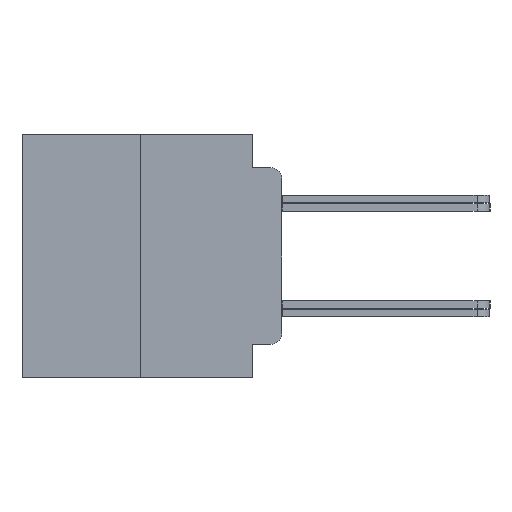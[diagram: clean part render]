
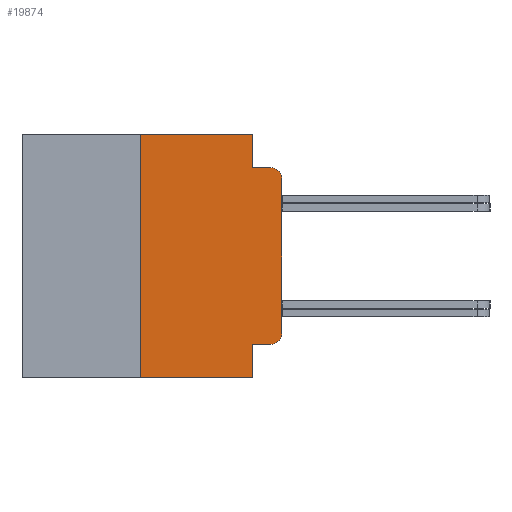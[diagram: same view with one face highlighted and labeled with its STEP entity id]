
A CAD part, left-side view. The second image highlights one B-rep face of the part: STEP entity #19874.
In plain terms, the highlighted planar face has unit normal (-1, 0, 0).
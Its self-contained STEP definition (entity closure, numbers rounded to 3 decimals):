
#359 = LINE ( 'NONE', #8364, #8279 ) ;
#578 = CARTESIAN_POINT ( 'NONE',  ( -75.603, 11.684, 5.486 ) ) ;
#1907 = CARTESIAN_POINT ( 'NONE',  ( -75.603, 6.35, -5.486 ) ) ;
#2023 = CARTESIAN_POINT ( 'NONE',  ( -75.603, 0., 3.467 ) ) ;
#2214 = PLANE ( 'NONE',  #18829 ) ;
#3100 = VERTEX_POINT ( 'NONE', #13580 ) ;
#3151 = DIRECTION ( 'NONE',  ( -1., 0., 0. ) ) ;
#3239 = CARTESIAN_POINT ( 'NONE',  ( -75.603, 0.508, 3.467 ) ) ;
#3272 = CARTESIAN_POINT ( 'NONE',  ( -75.603, 0., -3.467 ) ) ;
#3418 = LINE ( 'NONE', #21737, #19940 ) ;
#3507 = CARTESIAN_POINT ( 'NONE',  ( -75.603, 1.295, 3.975 ) ) ;
#3516 = LINE ( 'NONE', #10842, #7983 ) ;
#4163 = VERTEX_POINT ( 'NONE', #7434 ) ;
#4437 = ORIENTED_EDGE ( 'NONE', *, *, #12070, .T. ) ;
#5436 = DIRECTION ( 'NONE',  ( 0., 0., -1. ) ) ;
#5620 = VERTEX_POINT ( 'NONE', #2023 ) ;
#5876 = DIRECTION ( 'NONE',  ( 0., -1., 0. ) ) ;
#6233 = VECTOR ( 'NONE', #5876, 1000. ) ;
#6931 = CARTESIAN_POINT ( 'NONE',  ( -75.603, 11.684, 5.486 ) ) ;
#6961 = DIRECTION ( 'NONE',  ( 0., 0., 1. ) ) ;
#7434 = CARTESIAN_POINT ( 'NONE',  ( -75.603, 1.295, 5.486 ) ) ;
#7974 = EDGE_CURVE ( 'NONE', #4163, #26963, #23502, .T. ) ;
#7983 = VECTOR ( 'NONE', #6961, 1000. ) ;
#8014 = VERTEX_POINT ( 'NONE', #14384 ) ;
#8279 = VECTOR ( 'NONE', #26388, 1000. ) ;
#8364 = CARTESIAN_POINT ( 'NONE',  ( -75.603, 11.684, -5.486 ) ) ;
#8589 = VERTEX_POINT ( 'NONE', #22852 ) ;
#8658 = DIRECTION ( 'NONE',  ( 0., 0., 1. ) ) ;
#9074 = LINE ( 'NONE', #578, #13879 ) ;
#9078 = ORIENTED_EDGE ( 'NONE', *, *, #15068, .T. ) ;
#9659 = CARTESIAN_POINT ( 'NONE',  ( -75.603, 0.508, -3.467 ) ) ;
#9799 = EDGE_CURVE ( 'NONE', #5620, #3100, #20308, .T. ) ;
#10076 = CARTESIAN_POINT ( 'NONE',  ( -75.603, 1.295, 0. ) ) ;
#10661 = VERTEX_POINT ( 'NONE', #28404 ) ;
#10818 = VECTOR ( 'NONE', #8658, 1000. ) ;
#10842 = CARTESIAN_POINT ( 'NONE',  ( -75.603, 6.35, -5.486 ) ) ;
#11090 = VECTOR ( 'NONE', #11362, 1000. ) ;
#11362 = DIRECTION ( 'NONE',  ( 0., 0., -1. ) ) ;
#11541 = DIRECTION ( 'NONE',  ( 0., -1., 0. ) ) ;
#11876 = CARTESIAN_POINT ( 'NONE',  ( -75.603, 1.295, 3.975 ) ) ;
#12070 = EDGE_CURVE ( 'NONE', #10661, #8589, #3418, .T. ) ;
#12189 = LINE ( 'NONE', #26130, #10818 ) ;
#12424 = LINE ( 'NONE', #3507, #6233 ) ;
#12777 = DIRECTION ( 'NONE',  ( 0., -1., 0. ) ) ;
#13106 = ORIENTED_EDGE ( 'NONE', *, *, #9799, .T. ) ;
#13386 = ORIENTED_EDGE ( 'NONE', *, *, #18435, .F. ) ;
#13436 = VERTEX_POINT ( 'NONE', #17138 ) ;
#13580 = CARTESIAN_POINT ( 'NONE',  ( -75.603, 0.508, 3.975 ) ) ;
#13701 = EDGE_LOOP ( 'NONE', ( #4437, #24094, #9078, #13106, #21896, #23951, #22596, #27830, #27521, #13386 ) ) ;
#13879 = VECTOR ( 'NONE', #11541, 1000. ) ;
#13967 = DIRECTION ( 'NONE',  ( 0., 0., -1. ) ) ;
#14384 = CARTESIAN_POINT ( 'NONE',  ( -75.603, 6.35, 5.486 ) ) ;
#15051 = VERTEX_POINT ( 'NONE', #1907 ) ;
#15068 = EDGE_CURVE ( 'NONE', #18189, #5620, #12189, .T. ) ;
#15154 = VECTOR ( 'NONE', #26263, 1000. ) ;
#15923 = EDGE_CURVE ( 'NONE', #8014, #4163, #9074, .T. ) ;
#17138 = CARTESIAN_POINT ( 'NONE',  ( -75.603, 1.295, -5.486 ) ) ;
#17587 = DIRECTION ( 'NONE',  ( 1., 0., 0. ) ) ;
#17596 = EDGE_CURVE ( 'NONE', #8589, #18189, #20012, .T. ) ;
#18189 = VERTEX_POINT ( 'NONE', #3272 ) ;
#18435 = EDGE_CURVE ( 'NONE', #10661, #13436, #28308, .T. ) ;
#18829 = AXIS2_PLACEMENT_3D ( 'NONE', #6931, #17587, #22370 ) ;
#19520 = FACE_OUTER_BOUND ( 'NONE', #13701, .T. ) ;
#19561 = AXIS2_PLACEMENT_3D ( 'NONE', #3239, #3151, #5436 ) ;
#19874 = ADVANCED_FACE ( 'NONE', ( #19520 ), #2214, .F. ) ;
#19940 = VECTOR ( 'NONE', #12777, 1000. ) ;
#20012 = CIRCLE ( 'NONE', #24157, 0.508 ) ;
#20043 = CARTESIAN_POINT ( 'NONE',  ( -75.603, 1.295, 0. ) ) ;
#20308 = CIRCLE ( 'NONE', #19561, 0.508 ) ;
#21737 = CARTESIAN_POINT ( 'NONE',  ( -75.603, 1.295, -3.975 ) ) ;
#21896 = ORIENTED_EDGE ( 'NONE', *, *, #24012, .F. ) ;
#22370 = DIRECTION ( 'NONE',  ( 0., 0., -1. ) ) ;
#22596 = ORIENTED_EDGE ( 'NONE', *, *, #15923, .F. ) ;
#22852 = CARTESIAN_POINT ( 'NONE',  ( -75.603, 0.508, -3.975 ) ) ;
#23502 = LINE ( 'NONE', #20043, #11090 ) ;
#23690 = EDGE_CURVE ( 'NONE', #15051, #8014, #3516, .T. ) ;
#23951 = ORIENTED_EDGE ( 'NONE', *, *, #7974, .F. ) ;
#24012 = EDGE_CURVE ( 'NONE', #26963, #3100, #12424, .T. ) ;
#24094 = ORIENTED_EDGE ( 'NONE', *, *, #17596, .T. ) ;
#24157 = AXIS2_PLACEMENT_3D ( 'NONE', #9659, #27235, #13967 ) ;
#26130 = CARTESIAN_POINT ( 'NONE',  ( -75.603, 0., 5.486 ) ) ;
#26263 = DIRECTION ( 'NONE',  ( 0., 0., -1. ) ) ;
#26388 = DIRECTION ( 'NONE',  ( 0., -1., 0. ) ) ;
#26963 = VERTEX_POINT ( 'NONE', #11876 ) ;
#27235 = DIRECTION ( 'NONE',  ( -1., 0., 0. ) ) ;
#27521 = ORIENTED_EDGE ( 'NONE', *, *, #27780, .T. ) ;
#27780 = EDGE_CURVE ( 'NONE', #15051, #13436, #359, .T. ) ;
#27830 = ORIENTED_EDGE ( 'NONE', *, *, #23690, .F. ) ;
#28308 = LINE ( 'NONE', #10076, #15154 ) ;
#28404 = CARTESIAN_POINT ( 'NONE',  ( -75.603, 1.295, -3.975 ) ) ;
